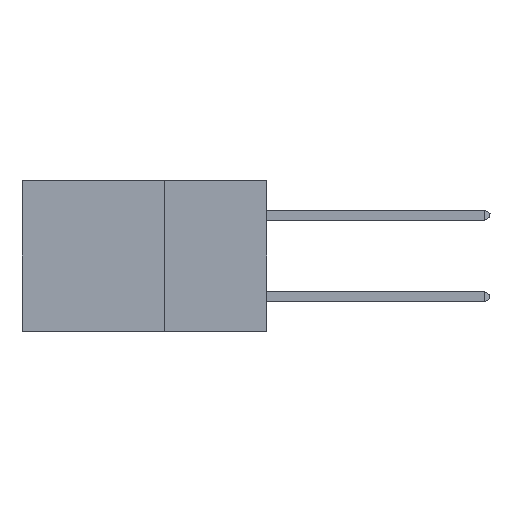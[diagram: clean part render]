
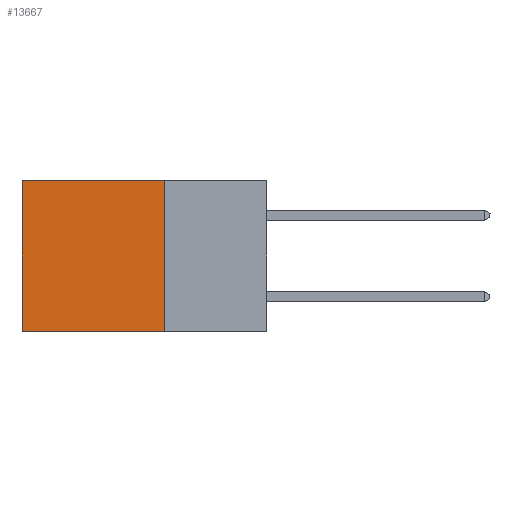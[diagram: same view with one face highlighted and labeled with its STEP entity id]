
A CAD part, left-side view. The second image highlights one B-rep face of the part: STEP entity #13667.
In plain terms, the highlighted planar face has unit normal (-1, 0, 0).
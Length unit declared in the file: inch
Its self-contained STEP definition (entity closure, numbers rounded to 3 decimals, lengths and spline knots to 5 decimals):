
#67 = LINE ( 'NONE', #28791, #25370 ) ;
#101 = EDGE_CURVE ( 'NONE', #28875, #25110, #67, .T. ) ;
#632 = VECTOR ( 'NONE', #24550, 39.37008 ) ;
#1071 = DIRECTION ( 'NONE',  ( 0., 1., 0. ) ) ;
#2109 = DIRECTION ( 'NONE',  ( 0., 1., 0. ) ) ;
#3094 = ORIENTED_EDGE ( 'NONE', *, *, #101, .F. ) ;
#3611 = CARTESIAN_POINT ( 'NONE',  ( 0.2875, 0.25, 0. ) ) ;
#4218 = CARTESIAN_POINT ( 'NONE',  ( 0.2875, 0.25, 0. ) ) ;
#4597 = CARTESIAN_POINT ( 'NONE',  ( 0.2875, 0.25, 0. ) ) ;
#8532 = EDGE_CURVE ( 'NONE', #40734, #25110, #9170, .T. ) ;
#9170 = LINE ( 'NONE', #25465, #16848 ) ;
#9580 = ORIENTED_EDGE ( 'NONE', *, *, #8532, .T. ) ;
#9798 = CARTESIAN_POINT ( 'NONE',  ( 0.2875, 0.25, 0. ) ) ;
#11003 = ORIENTED_EDGE ( 'NONE', *, *, #15630, .F. ) ;
#12766 = EDGE_LOOP ( 'NONE', ( #9580, #3094, #11003, #30412 ) ) ;
#12966 = PLANE ( 'NONE',  #34569 ) ;
#13667 = ADVANCED_FACE ( 'NONE', ( #41962 ), #12966, .F. ) ;
#15630 = EDGE_CURVE ( 'NONE', #41796, #28875, #22806, .T. ) ;
#16848 = VECTOR ( 'NONE', #28922, 39.37008 ) ;
#18901 = CARTESIAN_POINT ( 'NONE',  ( 0.2875, 0.25, -0.37 ) ) ;
#21559 = LINE ( 'NONE', #4218, #42132 ) ;
#22806 = LINE ( 'NONE', #3611, #632 ) ;
#24550 = DIRECTION ( 'NONE',  ( 0., 0., -1. ) ) ;
#25110 = VERTEX_POINT ( 'NONE', #35080 ) ;
#25370 = VECTOR ( 'NONE', #2109, 39.37008 ) ;
#25465 = CARTESIAN_POINT ( 'NONE',  ( 0.2875, 0.6, 0. ) ) ;
#28791 = CARTESIAN_POINT ( 'NONE',  ( 0.2875, 0.25, -0.37 ) ) ;
#28875 = VERTEX_POINT ( 'NONE', #18901 ) ;
#28922 = DIRECTION ( 'NONE',  ( 0., 0., -1. ) ) ;
#30412 = ORIENTED_EDGE ( 'NONE', *, *, #40928, .T. ) ;
#34569 = AXIS2_PLACEMENT_3D ( 'NONE', #9798, #36406, #36534 ) ;
#35080 = CARTESIAN_POINT ( 'NONE',  ( 0.2875, 0.6, -0.37 ) ) ;
#36406 = DIRECTION ( 'NONE',  ( 1., 0., 0. ) ) ;
#36534 = DIRECTION ( 'NONE',  ( 0., 0., -1. ) ) ;
#38967 = CARTESIAN_POINT ( 'NONE',  ( 0.2875, 0.6, 0. ) ) ;
#40734 = VERTEX_POINT ( 'NONE', #38967 ) ;
#40928 = EDGE_CURVE ( 'NONE', #41796, #40734, #21559, .T. ) ;
#41796 = VERTEX_POINT ( 'NONE', #4597 ) ;
#41962 = FACE_OUTER_BOUND ( 'NONE', #12766, .T. ) ;
#42132 = VECTOR ( 'NONE', #1071, 39.37008 ) ;
